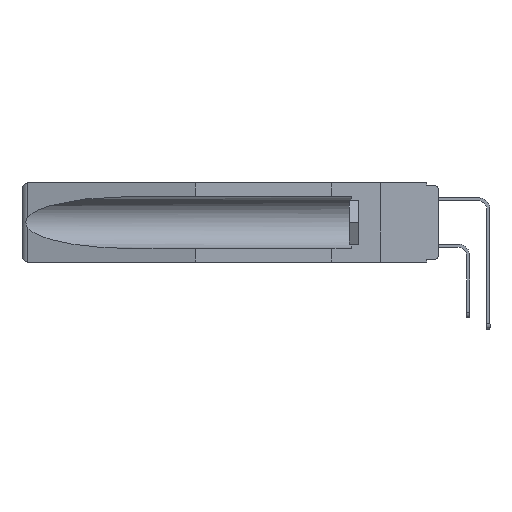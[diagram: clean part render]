
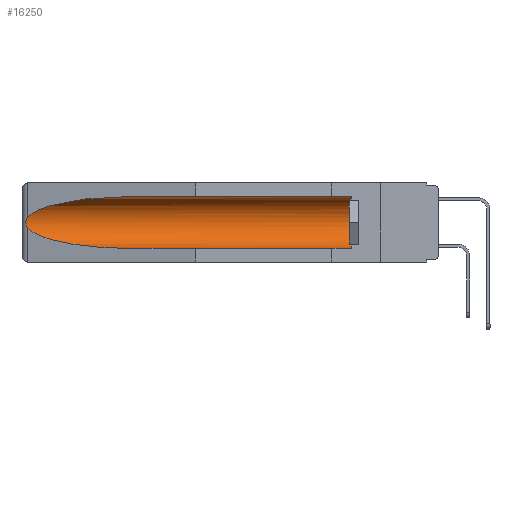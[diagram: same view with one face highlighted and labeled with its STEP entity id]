
A CAD part, left-side view. The second image highlights one B-rep face of the part: STEP entity #16250.
In plain terms, the highlighted cylindrical face has radius 2.857 mm (diameter 5.715 mm), a partial arc.
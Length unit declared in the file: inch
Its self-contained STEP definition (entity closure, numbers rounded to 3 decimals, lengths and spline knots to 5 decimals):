
#617 = CARTESIAN_POINT ( 'NONE',  ( 0.26537, 1.52718, -0.19328 ) ) ;
#868 = EDGE_CURVE ( 'NONE', #11721, #9723, #11282, .T. ) ;
#1756 = EDGE_LOOP ( 'NONE', ( #20210, #9636, #16172, #15816, #17890, #5225 ) ) ;
#2339 = EDGE_CURVE ( 'NONE', #11721, #23781, #23411, .T. ) ;
#2601 = CARTESIAN_POINT ( 'NONE',  ( 0.155, 1.07973, -0.284 ) ) ;
#3489 =( BOUNDED_CURVE ( )  B_SPLINE_CURVE ( 3, ( #24041, #22180, #12726, #2601 ),
 .UNSPECIFIED., .F., .F. ) 
 B_SPLINE_CURVE_WITH_KNOTS ( ( 4, 4 ),
 ( 0.1948, 1.5708 ),
 .UNSPECIFIED. ) 
 CURVE ( )  GEOMETRIC_REPRESENTATION_ITEM ( )  RATIONAL_B_SPLINE_CURVE ( ( 1., 0.848, 0.848, 1. ) ) 
 REPRESENTATION_ITEM ( '' )  );
#4169 = LINE ( 'NONE', #18638, #17836 ) ;
#4771 = DIRECTION ( 'NONE',  ( 0., 0., 1. ) ) ;
#5225 = ORIENTED_EDGE ( 'NONE', *, *, #8037, .T. ) ;
#5412 = CARTESIAN_POINT ( 'NONE',  ( 0.2673, 1.53269, -0.17917 ) ) ;
#5654 = CARTESIAN_POINT ( 'NONE',  ( 0.155, 0.126, -0.059 ) ) ;
#6345 = CARTESIAN_POINT ( 'NONE',  ( 0.26537, 1.52718, -0.14972 ) ) ;
#6789 = VERTEX_POINT ( 'NONE', #11534 ) ;
#7135 = DIRECTION ( 'NONE',  ( 0., -1., 0. ) ) ;
#7386 = CARTESIAN_POINT ( 'NONE',  ( 0.2675, 1.53308, -0.16763 ) ) ;
#7509 = CARTESIAN_POINT ( 'NONE',  ( 0.26597, 1.5296, -0.19026 ) ) ;
#8037 = EDGE_CURVE ( 'NONE', #9723, #24825, #4169, .T. ) ;
#8468 = FACE_OUTER_BOUND ( 'NONE', #1756, .T. ) ;
#9019 = EDGE_CURVE ( 'NONE', #24825, #6789, #18920, .T. ) ;
#9362 = AXIS2_PLACEMENT_3D ( 'NONE', #24494, #14518, #10577 ) ;
#9481 = CARTESIAN_POINT ( 'NONE',  ( 0.26537, 1.52718, -0.19328 ) ) ;
#9636 = ORIENTED_EDGE ( 'NONE', *, *, #18173, .T. ) ;
#9723 = VERTEX_POINT ( 'NONE', #5654 ) ;
#9748 = CARTESIAN_POINT ( 'NONE',  ( 0.2673, 1.5327, -0.16383 ) ) ;
#10577 = DIRECTION ( 'NONE',  ( 0., 0., 1. ) ) ;
#11282 = CIRCLE ( 'NONE', #20101, 0.1125 ) ;
#11534 = CARTESIAN_POINT ( 'NONE',  ( 0.26537, 1.52718, -0.14972 ) ) ;
#11721 = VERTEX_POINT ( 'NONE', #18465 ) ;
#12444 = DIRECTION ( 'NONE',  ( 0., 1., 0. ) ) ;
#12726 = CARTESIAN_POINT ( 'NONE',  ( 0.21114, 1.30732, -0.284 ) ) ;
#12825 = B_SPLINE_CURVE_WITH_KNOTS ( 'NONE', 3,
 ( #23668, #21814, #19476, #9748, #7386, #17370, #5412, #13418, #7509, #9481 ),
 .UNSPECIFIED., .F., .F.,
 ( 4, 2, 2, 2, 4 ),
 ( 0., 0.00029, 0.00058, 0.00087, 0.00117 ),
 .UNSPECIFIED. ) ;
#13418 = CARTESIAN_POINT ( 'NONE',  ( 0.26655, 1.53094, -0.18657 ) ) ;
#14518 = DIRECTION ( 'NONE',  ( 0., 1., 0. ) ) ;
#15816 = ORIENTED_EDGE ( 'NONE', *, *, #2339, .F. ) ;
#16172 = ORIENTED_EDGE ( 'NONE', *, *, #21158, .T. ) ;
#16250 = ADVANCED_FACE ( 'NONE', ( #8468 ), #16483, .F. ) ;
#16323 = CARTESIAN_POINT ( 'NONE',  ( 0.21114, 1.30732, -0.059 ) ) ;
#16483 = CYLINDRICAL_SURFACE ( 'NONE', #9362, 0.1125 ) ;
#17370 = CARTESIAN_POINT ( 'NONE',  ( 0.2675, 1.53308, -0.17534 ) ) ;
#17503 = CARTESIAN_POINT ( 'NONE',  ( 0.155, -0.30754, -0.284 ) ) ;
#17836 = VECTOR ( 'NONE', #12444, 39.37008 ) ;
#17890 = ORIENTED_EDGE ( 'NONE', *, *, #868, .T. ) ;
#18100 = CARTESIAN_POINT ( 'NONE',  ( 0.155, 1.07973, -0.059 ) ) ;
#18173 = EDGE_CURVE ( 'NONE', #6789, #18868, #12825, .T. ) ;
#18465 = CARTESIAN_POINT ( 'NONE',  ( 0.155, 0.126, -0.284 ) ) ;
#18638 = CARTESIAN_POINT ( 'NONE',  ( 0.155, -0.30754, -0.059 ) ) ;
#18710 = CARTESIAN_POINT ( 'NONE',  ( 0.155, 0.126, -0.1715 ) ) ;
#18868 = VERTEX_POINT ( 'NONE', #617 ) ;
#18920 =( BOUNDED_CURVE ( )  B_SPLINE_CURVE ( 3, ( #24475, #16323, #24341, #6345 ),
 .UNSPECIFIED., .F., .F. ) 
 B_SPLINE_CURVE_WITH_KNOTS ( ( 4, 4 ),
 ( 4.71239, 6.08839 ),
 .UNSPECIFIED. ) 
 CURVE ( )  GEOMETRIC_REPRESENTATION_ITEM ( )  RATIONAL_B_SPLINE_CURVE ( ( 1., 0.848, 0.848, 1. ) ) 
 REPRESENTATION_ITEM ( '' )  );
#19476 = CARTESIAN_POINT ( 'NONE',  ( 0.26654, 1.53092, -0.15636 ) ) ;
#20101 = AXIS2_PLACEMENT_3D ( 'NONE', #18710, #7135, #4771 ) ;
#20210 = ORIENTED_EDGE ( 'NONE', *, *, #9019, .T. ) ;
#20293 = CARTESIAN_POINT ( 'NONE',  ( 0.155, 1.07973, -0.284 ) ) ;
#21158 = EDGE_CURVE ( 'NONE', #18868, #23781, #3489, .T. ) ;
#21814 = CARTESIAN_POINT ( 'NONE',  ( 0.26597, 1.52961, -0.15275 ) ) ;
#21964 = VECTOR ( 'NONE', #25510, 39.37008 ) ;
#22180 = CARTESIAN_POINT ( 'NONE',  ( 0.25451, 1.48313, -0.24835 ) ) ;
#23411 = LINE ( 'NONE', #17503, #21964 ) ;
#23668 = CARTESIAN_POINT ( 'NONE',  ( 0.26537, 1.52718, -0.14972 ) ) ;
#23781 = VERTEX_POINT ( 'NONE', #20293 ) ;
#24041 = CARTESIAN_POINT ( 'NONE',  ( 0.26537, 1.52718, -0.19328 ) ) ;
#24341 = CARTESIAN_POINT ( 'NONE',  ( 0.25451, 1.48313, -0.09465 ) ) ;
#24475 = CARTESIAN_POINT ( 'NONE',  ( 0.155, 1.07973, -0.059 ) ) ;
#24494 = CARTESIAN_POINT ( 'NONE',  ( 0.155, -0.30754, -0.1715 ) ) ;
#24825 = VERTEX_POINT ( 'NONE', #18100 ) ;
#25510 = DIRECTION ( 'NONE',  ( 0., 1., 0. ) ) ;
